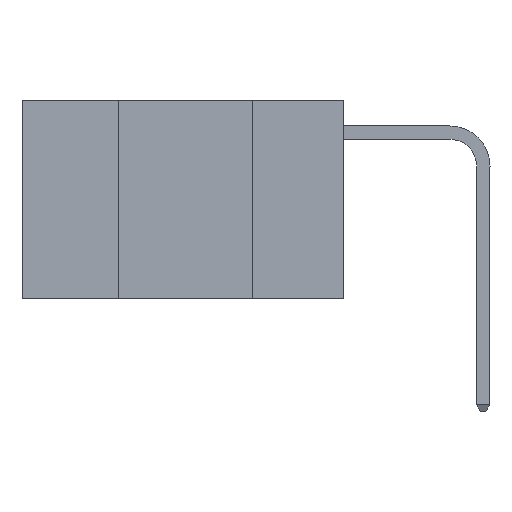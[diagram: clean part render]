
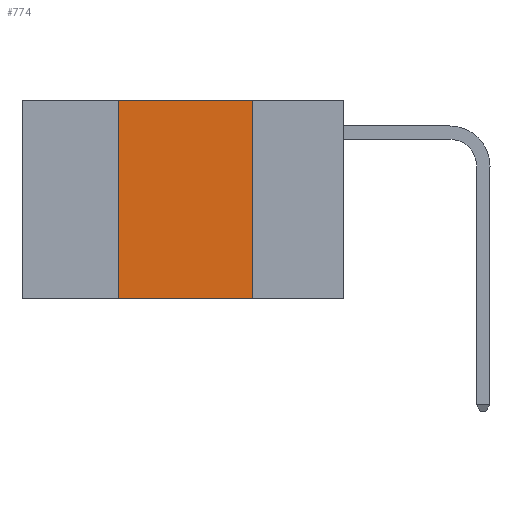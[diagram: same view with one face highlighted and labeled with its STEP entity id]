
A CAD part, left-side view. The second image highlights one B-rep face of the part: STEP entity #774.
In plain terms, the highlighted planar face has unit normal (-1, 0, 0).
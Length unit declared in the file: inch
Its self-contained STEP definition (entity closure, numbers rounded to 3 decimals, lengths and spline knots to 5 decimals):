
#774 = ADVANCED_FACE ( 'NONE', ( #14601 ), #3397, .F. ) ;
#1250 = LINE ( 'NONE', #13671, #8103 ) ;
#1872 = CARTESIAN_POINT ( 'NONE',  ( 0., 0.42, 0. ) ) ;
#2248 = DIRECTION ( 'NONE',  ( 0., 0., -1. ) ) ;
#2521 = ORIENTED_EDGE ( 'NONE', *, *, #3078, .F. ) ;
#3078 = EDGE_CURVE ( 'NONE', #3290, #5336, #14338, .T. ) ;
#3290 = VERTEX_POINT ( 'NONE', #1872 ) ;
#3397 = PLANE ( 'NONE',  #11038 ) ;
#3474 = CARTESIAN_POINT ( 'NONE',  ( 0., 0.17, -0.37 ) ) ;
#3948 = VECTOR ( 'NONE', #11264, 39.37008 ) ;
#4098 = VERTEX_POINT ( 'NONE', #3474 ) ;
#4493 = VERTEX_POINT ( 'NONE', #5419 ) ;
#5336 = VERTEX_POINT ( 'NONE', #15655 ) ;
#5419 = CARTESIAN_POINT ( 'NONE',  ( 0., 0.42, -0.37 ) ) ;
#5727 = ORIENTED_EDGE ( 'NONE', *, *, #11402, .F. ) ;
#6254 = VECTOR ( 'NONE', #7172, 39.37008 ) ;
#7172 = DIRECTION ( 'NONE',  ( 0., -1., 0. ) ) ;
#8073 = DIRECTION ( 'NONE',  ( 0., 0., 1. ) ) ;
#8103 = VECTOR ( 'NONE', #10106, 39.37008 ) ;
#8585 = ORIENTED_EDGE ( 'NONE', *, *, #12192, .F. ) ;
#9499 = DIRECTION ( 'NONE',  ( 1., 0., 0. ) ) ;
#10027 = CARTESIAN_POINT ( 'NONE',  ( 0., 0.6, 0. ) ) ;
#10106 = DIRECTION ( 'NONE',  ( 0., 0., -1. ) ) ;
#10552 = EDGE_CURVE ( 'NONE', #4493, #4098, #12718, .T. ) ;
#11038 = AXIS2_PLACEMENT_3D ( 'NONE', #11897, #9499, #2248 ) ;
#11264 = DIRECTION ( 'NONE',  ( 0., -1., 0. ) ) ;
#11402 = EDGE_CURVE ( 'NONE', #4493, #3290, #14676, .T. ) ;
#11636 = EDGE_LOOP ( 'NONE', ( #8585, #2521, #5727, #15648 ) ) ;
#11897 = CARTESIAN_POINT ( 'NONE',  ( 0., 0.6, 0. ) ) ;
#11934 = VECTOR ( 'NONE', #8073, 39.37008 ) ;
#12192 = EDGE_CURVE ( 'NONE', #5336, #4098, #1250, .T. ) ;
#12718 = LINE ( 'NONE', #15553, #6254 ) ;
#13671 = CARTESIAN_POINT ( 'NONE',  ( 0., 0.17, 0. ) ) ;
#14338 = LINE ( 'NONE', #10027, #3948 ) ;
#14601 = FACE_OUTER_BOUND ( 'NONE', #11636, .T. ) ;
#14676 = LINE ( 'NONE', #15225, #11934 ) ;
#15225 = CARTESIAN_POINT ( 'NONE',  ( 0., 0.42, 0. ) ) ;
#15553 = CARTESIAN_POINT ( 'NONE',  ( 0., 0.6, -0.37 ) ) ;
#15648 = ORIENTED_EDGE ( 'NONE', *, *, #10552, .T. ) ;
#15655 = CARTESIAN_POINT ( 'NONE',  ( 0., 0.17, 0. ) ) ;
